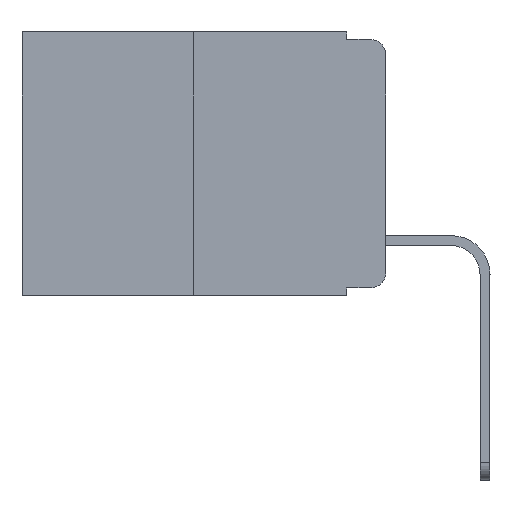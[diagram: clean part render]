
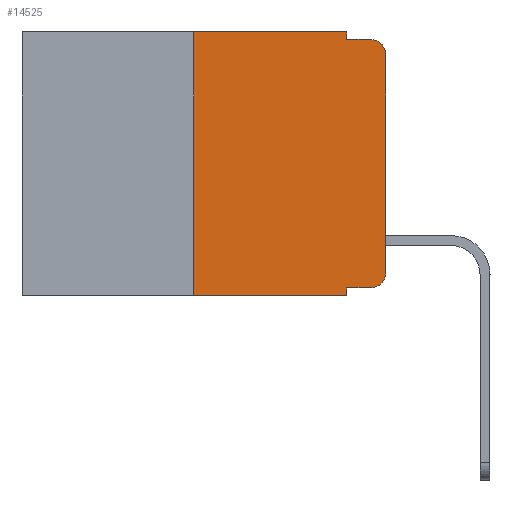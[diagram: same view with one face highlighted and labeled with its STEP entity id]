
A CAD part, left-side view. The second image highlights one B-rep face of the part: STEP entity #14525.
In plain terms, the highlighted planar face has unit normal (-1, 0, 0).
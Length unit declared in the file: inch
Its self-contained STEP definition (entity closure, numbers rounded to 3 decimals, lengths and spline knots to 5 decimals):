
#386 = DIRECTION ( 'NONE',  ( 1., 0., 0. ) ) ;
#606 = PLANE ( 'NONE',  #21876 ) ;
#956 = CARTESIAN_POINT ( 'NONE',  ( 0., 0., 0. ) ) ;
#1081 = DIRECTION ( 'NONE',  ( 0., -1., 0. ) ) ;
#1627 = VERTEX_POINT ( 'NONE', #9377 ) ;
#1679 = CARTESIAN_POINT ( 'NONE',  ( 0., 0.051, -0.01 ) ) ;
#1999 = VERTEX_POINT ( 'NONE', #8281 ) ;
#2374 = LINE ( 'NONE', #2653, #15348 ) ;
#2437 = CARTESIAN_POINT ( 'NONE',  ( 0., 0.051, -0.333 ) ) ;
#2479 = LINE ( 'NONE', #12497, #15157 ) ;
#2653 = CARTESIAN_POINT ( 'NONE',  ( 0., 0.473, -0.343 ) ) ;
#2679 = CARTESIAN_POINT ( 'NONE',  ( 0., 0., -0.03 ) ) ;
#3204 = LINE ( 'NONE', #3800, #21416 ) ;
#3622 = ORIENTED_EDGE ( 'NONE', *, *, #7237, .F. ) ;
#3800 = CARTESIAN_POINT ( 'NONE',  ( 0., 0.25, 0. ) ) ;
#3811 = LINE ( 'NONE', #12907, #18660 ) ;
#4760 = DIRECTION ( 'NONE',  ( 0., -1., 0. ) ) ;
#5434 = DIRECTION ( 'NONE',  ( 0., 0., -1. ) ) ;
#5501 = VERTEX_POINT ( 'NONE', #10642 ) ;
#5838 = CARTESIAN_POINT ( 'NONE',  ( 0., 0.02, -0.313 ) ) ;
#6330 = DIRECTION ( 'NONE',  ( 0., 0., 1. ) ) ;
#6350 = EDGE_CURVE ( 'NONE', #5501, #18951, #2374, .T. ) ;
#6878 = EDGE_CURVE ( 'NONE', #5501, #22834, #3204, .T. ) ;
#7075 = CARTESIAN_POINT ( 'NONE',  ( 0., 0.473, 0. ) ) ;
#7237 = EDGE_CURVE ( 'NONE', #22834, #1999, #15902, .T. ) ;
#7640 = CARTESIAN_POINT ( 'NONE',  ( 0., 0.473, 0. ) ) ;
#7964 = ORIENTED_EDGE ( 'NONE', *, *, #21131, .T. ) ;
#8125 = LINE ( 'NONE', #956, #12001 ) ;
#8281 = CARTESIAN_POINT ( 'NONE',  ( 0., 0.051, 0. ) ) ;
#8536 = ORIENTED_EDGE ( 'NONE', *, *, #15437, .T. ) ;
#9018 = CARTESIAN_POINT ( 'NONE',  ( 0., 0.02, -0.01 ) ) ;
#9167 = CIRCLE ( 'NONE', #21224, 0.02 ) ;
#9327 = VERTEX_POINT ( 'NONE', #9018 ) ;
#9377 = CARTESIAN_POINT ( 'NONE',  ( 0., 0., -0.313 ) ) ;
#9381 = CARTESIAN_POINT ( 'NONE',  ( 0., 0.051, -0.01 ) ) ;
#10355 = EDGE_CURVE ( 'NONE', #16303, #9327, #15386, .T. ) ;
#10642 = CARTESIAN_POINT ( 'NONE',  ( 0., 0.25, -0.343 ) ) ;
#10647 = ORIENTED_EDGE ( 'NONE', *, *, #18909, .F. ) ;
#10874 = DIRECTION ( 'NONE',  ( 0., 0., -1. ) ) ;
#10909 = DIRECTION ( 'NONE',  ( 0., 0., -1. ) ) ;
#10953 = DIRECTION ( 'NONE',  ( -1., 0., 0. ) ) ;
#10956 = DIRECTION ( 'NONE',  ( 0., -1., 0. ) ) ;
#11317 = DIRECTION ( 'NONE',  ( -1., 0., 0. ) ) ;
#11458 = DIRECTION ( 'NONE',  ( 0., 0., -1. ) ) ;
#11762 = VECTOR ( 'NONE', #19395, 39.37008 ) ;
#12001 = VECTOR ( 'NONE', #6330, 39.37008 ) ;
#12078 = VERTEX_POINT ( 'NONE', #2679 ) ;
#12497 = CARTESIAN_POINT ( 'NONE',  ( 0., 0.051, 0. ) ) ;
#12907 = CARTESIAN_POINT ( 'NONE',  ( 0., 0.051, 0. ) ) ;
#12968 = DIRECTION ( 'NONE',  ( 0., 0., -1. ) ) ;
#13106 = EDGE_CURVE ( 'NONE', #1627, #12078, #8125, .T. ) ;
#13121 = CARTESIAN_POINT ( 'NONE',  ( 0., 0.051, -0.333 ) ) ;
#14043 = VECTOR ( 'NONE', #10956, 39.37008 ) ;
#14287 = DIRECTION ( 'NONE',  ( 0., 0., 1. ) ) ;
#14525 = ADVANCED_FACE ( 'NONE', ( #20766 ), #606, .F. ) ;
#14704 = ORIENTED_EDGE ( 'NONE', *, *, #6878, .F. ) ;
#14735 = LINE ( 'NONE', #2437, #21645 ) ;
#15157 = VECTOR ( 'NONE', #10909, 39.37008 ) ;
#15348 = VECTOR ( 'NONE', #4760, 39.37008 ) ;
#15386 = LINE ( 'NONE', #9381, #14043 ) ;
#15437 = EDGE_CURVE ( 'NONE', #16013, #21870, #14735, .T. ) ;
#15458 = ORIENTED_EDGE ( 'NONE', *, *, #6350, .T. ) ;
#15902 = LINE ( 'NONE', #7075, #11762 ) ;
#16013 = VERTEX_POINT ( 'NONE', #13121 ) ;
#16133 = ORIENTED_EDGE ( 'NONE', *, *, #21328, .F. ) ;
#16204 = CIRCLE ( 'NONE', #22737, 0.02 ) ;
#16259 = CARTESIAN_POINT ( 'NONE',  ( 0., 0.051, -0.343 ) ) ;
#16303 = VERTEX_POINT ( 'NONE', #1679 ) ;
#18006 = EDGE_CURVE ( 'NONE', #21870, #1627, #9167, .T. ) ;
#18590 = ORIENTED_EDGE ( 'NONE', *, *, #10355, .F. ) ;
#18660 = VECTOR ( 'NONE', #5434, 39.37008 ) ;
#18909 = EDGE_CURVE ( 'NONE', #1999, #16303, #2479, .T. ) ;
#18951 = VERTEX_POINT ( 'NONE', #16259 ) ;
#19264 = ORIENTED_EDGE ( 'NONE', *, *, #13106, .T. ) ;
#19395 = DIRECTION ( 'NONE',  ( 0., -1., 0. ) ) ;
#19473 = CARTESIAN_POINT ( 'NONE',  ( 0., 0.02, -0.03 ) ) ;
#19810 = CARTESIAN_POINT ( 'NONE',  ( 0., 0.25, 0. ) ) ;
#20422 = ORIENTED_EDGE ( 'NONE', *, *, #18006, .T. ) ;
#20766 = FACE_OUTER_BOUND ( 'NONE', #22653, .T. ) ;
#21003 = CARTESIAN_POINT ( 'NONE',  ( 0., 0.02, -0.333 ) ) ;
#21131 = EDGE_CURVE ( 'NONE', #12078, #9327, #16204, .T. ) ;
#21224 = AXIS2_PLACEMENT_3D ( 'NONE', #5838, #11317, #11458 ) ;
#21328 = EDGE_CURVE ( 'NONE', #16013, #18951, #3811, .T. ) ;
#21416 = VECTOR ( 'NONE', #14287, 39.37008 ) ;
#21645 = VECTOR ( 'NONE', #1081, 39.37008 ) ;
#21870 = VERTEX_POINT ( 'NONE', #21003 ) ;
#21876 = AXIS2_PLACEMENT_3D ( 'NONE', #7640, #386, #12968 ) ;
#22653 = EDGE_LOOP ( 'NONE', ( #19264, #7964, #18590, #10647, #3622, #14704, #15458, #16133, #8536, #20422 ) ) ;
#22737 = AXIS2_PLACEMENT_3D ( 'NONE', #19473, #10953, #10874 ) ;
#22834 = VERTEX_POINT ( 'NONE', #19810 ) ;
